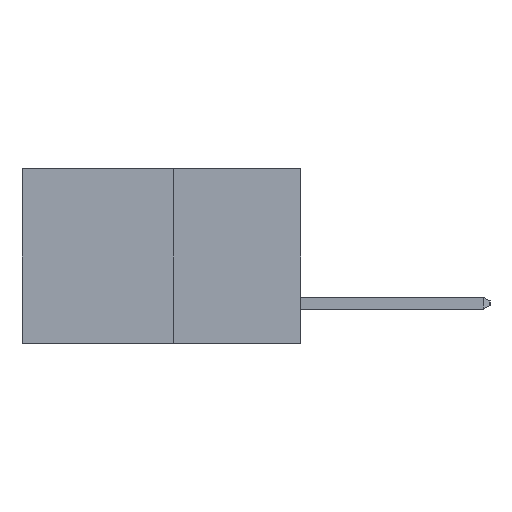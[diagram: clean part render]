
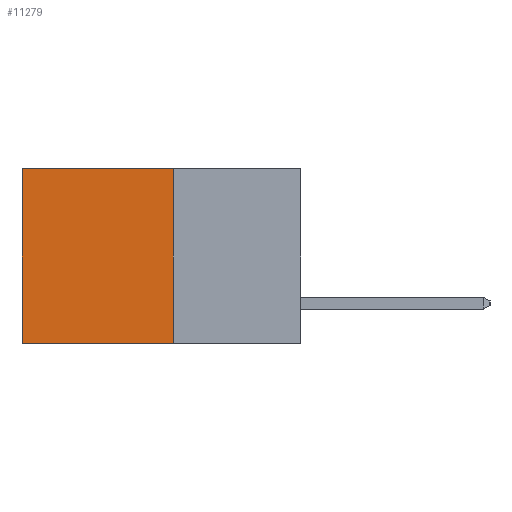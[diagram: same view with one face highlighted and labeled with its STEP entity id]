
A CAD part, left-side view. The second image highlights one B-rep face of the part: STEP entity #11279.
In plain terms, the highlighted planar face has unit normal (-1, 0, 0).
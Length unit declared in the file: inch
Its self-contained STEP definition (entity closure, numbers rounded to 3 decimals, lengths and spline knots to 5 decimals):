
#6 = CARTESIAN_POINT ( 'NONE',  ( 0.277, 0.27, 0. ) ) ;
#277 = EDGE_CURVE ( 'NONE', #2103, #12846, #3895, .T. ) ;
#956 = DIRECTION ( 'NONE',  ( 0., 1., 0. ) ) ;
#1348 = ORIENTED_EDGE ( 'NONE', *, *, #277, .F. ) ;
#1452 = VERTEX_POINT ( 'NONE', #8376 ) ;
#1499 = CARTESIAN_POINT ( 'NONE',  ( 0.277, 0.27, -0.37 ) ) ;
#2103 = VERTEX_POINT ( 'NONE', #8049 ) ;
#3154 = EDGE_LOOP ( 'NONE', ( #7745, #1348, #3460, #12860 ) ) ;
#3460 = ORIENTED_EDGE ( 'NONE', *, *, #7323, .F. ) ;
#3503 = CARTESIAN_POINT ( 'NONE',  ( 0.277, 0.59, 0. ) ) ;
#3584 = VECTOR ( 'NONE', #12033, 39.37008 ) ;
#3895 = LINE ( 'NONE', #11995, #3584 ) ;
#5671 = DIRECTION ( 'NONE',  ( 0., 0., -1. ) ) ;
#5676 = CARTESIAN_POINT ( 'NONE',  ( 0.277, 0.59, -0.37 ) ) ;
#5954 = DIRECTION ( 'NONE',  ( 1., 0., 0. ) ) ;
#6272 = VERTEX_POINT ( 'NONE', #3503 ) ;
#6361 = FACE_OUTER_BOUND ( 'NONE', #3154, .T. ) ;
#6466 = EDGE_CURVE ( 'NONE', #1452, #6272, #11942, .T. ) ;
#6617 = LINE ( 'NONE', #1499, #8943 ) ;
#6957 = VECTOR ( 'NONE', #956, 39.37008 ) ;
#7323 = EDGE_CURVE ( 'NONE', #1452, #2103, #6617, .T. ) ;
#7745 = ORIENTED_EDGE ( 'NONE', *, *, #8382, .T. ) ;
#8049 = CARTESIAN_POINT ( 'NONE',  ( 0.277, 0.27, -0.37 ) ) ;
#8374 = DIRECTION ( 'NONE',  ( 0., 0., -1. ) ) ;
#8376 = CARTESIAN_POINT ( 'NONE',  ( 0.277, 0.27, 0. ) ) ;
#8382 = EDGE_CURVE ( 'NONE', #6272, #12846, #9062, .T. ) ;
#8899 = PLANE ( 'NONE',  #9557 ) ;
#8943 = VECTOR ( 'NONE', #8374, 39.37008 ) ;
#9062 = LINE ( 'NONE', #5676, #11720 ) ;
#9557 = AXIS2_PLACEMENT_3D ( 'NONE', #11921, #5954, #12909 ) ;
#11279 = ADVANCED_FACE ( 'NONE', ( #6361 ), #8899, .F. ) ;
#11720 = VECTOR ( 'NONE', #5671, 39.37008 ) ;
#11792 = CARTESIAN_POINT ( 'NONE',  ( 0.277, 0.59, -0.37 ) ) ;
#11921 = CARTESIAN_POINT ( 'NONE',  ( 0.277, 0.27, -0.37 ) ) ;
#11942 = LINE ( 'NONE', #6, #6957 ) ;
#11995 = CARTESIAN_POINT ( 'NONE',  ( 0.277, 0.27, -0.37 ) ) ;
#12033 = DIRECTION ( 'NONE',  ( 0., 1., 0. ) ) ;
#12846 = VERTEX_POINT ( 'NONE', #11792 ) ;
#12860 = ORIENTED_EDGE ( 'NONE', *, *, #6466, .T. ) ;
#12909 = DIRECTION ( 'NONE',  ( 0., 0., -1. ) ) ;
